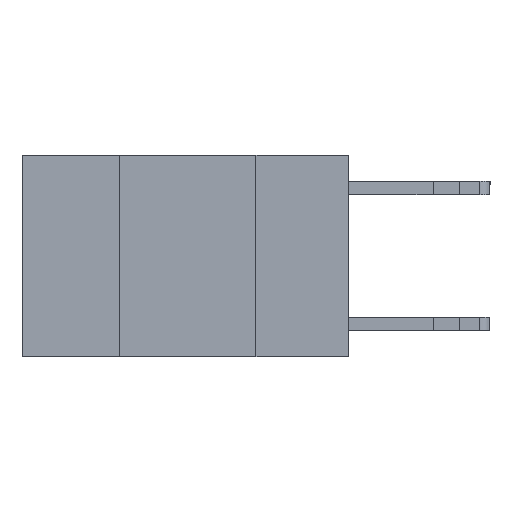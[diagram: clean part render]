
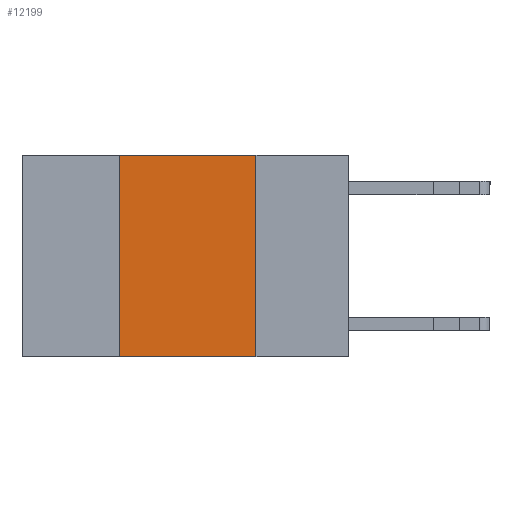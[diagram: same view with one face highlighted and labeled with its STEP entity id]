
A CAD part, left-side view. The second image highlights one B-rep face of the part: STEP entity #12199.
In plain terms, the highlighted planar face has unit normal (-1, 0, 0).
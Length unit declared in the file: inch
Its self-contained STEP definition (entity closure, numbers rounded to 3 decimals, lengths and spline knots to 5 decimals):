
#495 = EDGE_CURVE ( 'NONE', #17297, #26221, #19651, .T. ) ;
#519 = FACE_OUTER_BOUND ( 'NONE', #15490, .T. ) ;
#1151 = EDGE_CURVE ( 'NONE', #17297, #8529, #26278, .T. ) ;
#1331 = ORIENTED_EDGE ( 'NONE', *, *, #1151, .T. ) ;
#1871 = LINE ( 'NONE', #13993, #22656 ) ;
#2743 = ORIENTED_EDGE ( 'NONE', *, *, #19177, .F. ) ;
#3183 = CARTESIAN_POINT ( 'NONE',  ( 0., 0.6, -0.37 ) ) ;
#3837 = DIRECTION ( 'NONE',  ( 0., 0., -1. ) ) ;
#3887 = ORIENTED_EDGE ( 'NONE', *, *, #10569, .F. ) ;
#4868 = DIRECTION ( 'NONE',  ( 0., -1., 0. ) ) ;
#6529 = CARTESIAN_POINT ( 'NONE',  ( 0., 0.6, 0. ) ) ;
#6535 = VERTEX_POINT ( 'NONE', #17400 ) ;
#7505 = PLANE ( 'NONE',  #27412 ) ;
#7963 = VECTOR ( 'NONE', #25989, 39.37008 ) ;
#8529 = VERTEX_POINT ( 'NONE', #13830 ) ;
#10569 = EDGE_CURVE ( 'NONE', #26221, #6535, #17014, .T. ) ;
#11473 = VECTOR ( 'NONE', #4868, 39.37008 ) ;
#12199 = ADVANCED_FACE ( 'NONE', ( #519 ), #7505, .F. ) ;
#13755 = CARTESIAN_POINT ( 'NONE',  ( 0., 0.42, 0. ) ) ;
#13830 = CARTESIAN_POINT ( 'NONE',  ( 0., 0.17, -0.37 ) ) ;
#13993 = CARTESIAN_POINT ( 'NONE',  ( 0., 0.17, 0. ) ) ;
#15490 = EDGE_LOOP ( 'NONE', ( #2743, #3887, #26614, #1331 ) ) ;
#16559 = VECTOR ( 'NONE', #16740, 39.37008 ) ;
#16740 = DIRECTION ( 'NONE',  ( 0., -1., 0. ) ) ;
#17014 = LINE ( 'NONE', #6529, #16559 ) ;
#17297 = VERTEX_POINT ( 'NONE', #22386 ) ;
#17400 = CARTESIAN_POINT ( 'NONE',  ( 0., 0.17, 0. ) ) ;
#17572 = CARTESIAN_POINT ( 'NONE',  ( 0., 0.42, 0. ) ) ;
#19177 = EDGE_CURVE ( 'NONE', #6535, #8529, #1871, .T. ) ;
#19651 = LINE ( 'NONE', #17572, #7963 ) ;
#19789 = DIRECTION ( 'NONE',  ( 0., 0., -1. ) ) ;
#22386 = CARTESIAN_POINT ( 'NONE',  ( 0., 0.42, -0.37 ) ) ;
#22656 = VECTOR ( 'NONE', #3837, 39.37008 ) ;
#24009 = DIRECTION ( 'NONE',  ( 1., 0., 0. ) ) ;
#25989 = DIRECTION ( 'NONE',  ( 0., 0., 1. ) ) ;
#26116 = CARTESIAN_POINT ( 'NONE',  ( 0., 0.6, 0. ) ) ;
#26221 = VERTEX_POINT ( 'NONE', #13755 ) ;
#26278 = LINE ( 'NONE', #3183, #11473 ) ;
#26614 = ORIENTED_EDGE ( 'NONE', *, *, #495, .F. ) ;
#27412 = AXIS2_PLACEMENT_3D ( 'NONE', #26116, #24009, #19789 ) ;
